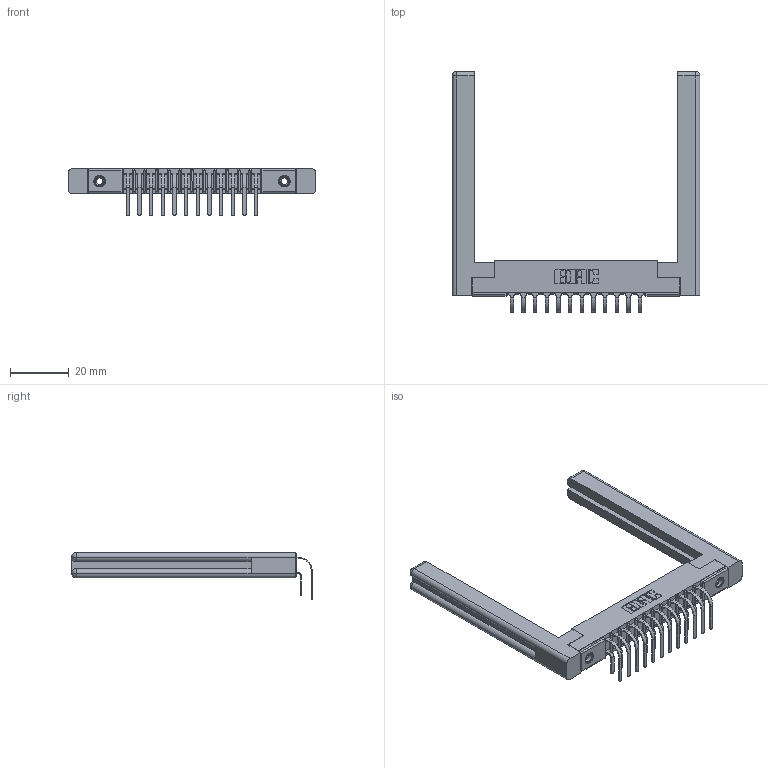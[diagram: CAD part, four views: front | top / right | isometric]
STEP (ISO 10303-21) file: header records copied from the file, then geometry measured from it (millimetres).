
FILE_DESCRIPTION (( 'STEP AP203' ), '1' );
FILE_NAME ('357-024-559-258.STEP', '2022-07-09T00:15:54', ( '' ), ( '' ), 'SwSTEP 2.0', 'SolidWorks 2020', '' );
FILE_SCHEMA (( 'CONFIG_CONTROL_DESIGN' ));
Length unit declared in the file: inch
Products named in the file (6): 345-250-001_345-250-001-102; 307-220-058; 307 Part_.156 Dia Mounting Holes; 357-024-559-258; 307-290-001_559 - 2 (Single); 307-290-001_558 559 - 1 (Single)
Assembly tree (29 placements, depth 2):
  357-024-559-258
    307 Part_.156 Dia Mounting Holes
    307-290-001_558 559 - 1 (Single)  x12
    307-290-001_559 - 2 (Single)  x12
    307-220-058  x2
    345-250-001_345-250-001-102  x2
Bounding box: 84.18 x 81.83 x 16.08 mm (x, y, z)
Volume: 13284 mm3; surface area: 14956.5 mm2
Topology: 29 solids, 29 shells, 1473 faces, 4085 edges, 2642 vertices
Faces by surface type: plane 946, cylinder 477, sphere 26, torus 12, cone 12
Entity records: 18450 total; most frequent: CARTESIAN_POINT 3049, ORIENTED_EDGE 2960, DIRECTION 2956, EDGE_CURVE 1480, LINE 1118, VECTOR 1118, VERTEX_POINT 958, AXIS2_PLACEMENT_3D 919
